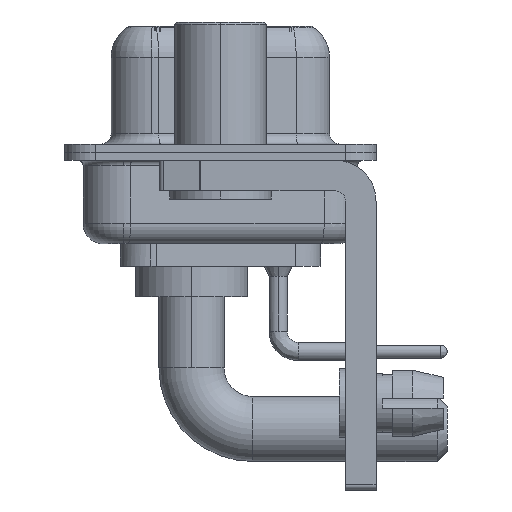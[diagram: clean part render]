
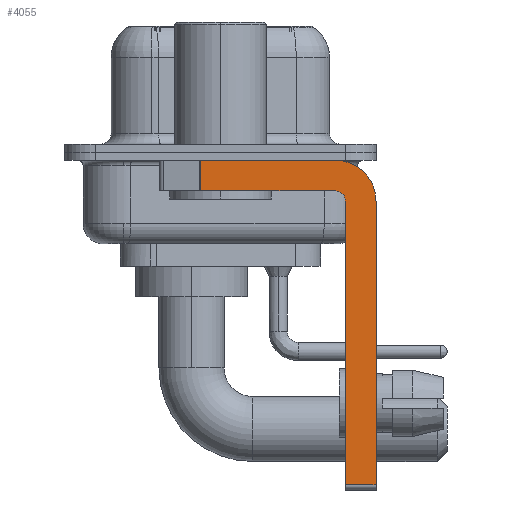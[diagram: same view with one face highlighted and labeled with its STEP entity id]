
A CAD part, left-side view. The second image highlights one B-rep face of the part: STEP entity #4055.
In plain terms, the highlighted planar face has unit normal (-1, 0, 0).
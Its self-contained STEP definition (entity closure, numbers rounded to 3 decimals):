
#403 = CARTESIAN_POINT ( 'NONE',  ( -2.9, -6.15, -16.6 ) ) ;
#712 = LINE ( 'NONE', #10209, #11654 ) ;
#1400 = CIRCLE ( 'NONE', #18189, 2. ) ;
#1860 = CARTESIAN_POINT ( 'NONE',  ( -2.9, 0.978, -0.4 ) ) ;
#1988 = LINE ( 'NONE', #25320, #6661 ) ;
#2259 = VERTEX_POINT ( 'NONE', #6362 ) ;
#2301 = EDGE_CURVE ( 'NONE', #12486, #19635, #712, .T. ) ;
#2708 = DIRECTION ( 'NONE',  ( -1., 0., 0. ) ) ;
#2727 = LINE ( 'NONE', #24270, #3816 ) ;
#2731 = PLANE ( 'NONE',  #23959 ) ;
#2754 = ORIENTED_EDGE ( 'NONE', *, *, #25264, .F. ) ;
#3429 = EDGE_CURVE ( 'NONE', #24635, #15286, #1400, .T. ) ;
#3816 = VECTOR ( 'NONE', #10178, 1000. ) ;
#4055 = ADVANCED_FACE ( 'NONE', ( #19576 ), #2731, .F. ) ;
#5858 = CARTESIAN_POINT ( 'NONE',  ( -2.9, -5.65, -2.4 ) ) ;
#6362 = CARTESIAN_POINT ( 'NONE',  ( -2.9, -5.65, -1.9 ) ) ;
#6596 = EDGE_CURVE ( 'NONE', #2259, #19635, #2727, .T. ) ;
#6661 = VECTOR ( 'NONE', #11464, 1000. ) ;
#7591 = EDGE_LOOP ( 'NONE', ( #2754, #23957, #9406, #24365, #22750, #23461, #15998, #7898 ) ) ;
#7898 = ORIENTED_EDGE ( 'NONE', *, *, #3429, .F. ) ;
#8478 = LINE ( 'NONE', #403, #12207 ) ;
#8719 = DIRECTION ( 'NONE',  ( 0., 0., 1. ) ) ;
#9117 = VERTEX_POINT ( 'NONE', #19627 ) ;
#9406 = ORIENTED_EDGE ( 'NONE', *, *, #6596, .F. ) ;
#9830 = DIRECTION ( 'NONE',  ( 0., 0., -1. ) ) ;
#10178 = DIRECTION ( 'NONE',  ( 0., 1., 0. ) ) ;
#10209 = CARTESIAN_POINT ( 'NONE',  ( -2.9, 0.978, -1.9 ) ) ;
#11200 = LINE ( 'NONE', #16843, #11901 ) ;
#11261 = CIRCLE ( 'NONE', #17821, 0.5 ) ;
#11272 = DIRECTION ( 'NONE',  ( 1., 0., 0. ) ) ;
#11388 = CARTESIAN_POINT ( 'NONE',  ( -2.9, -5.65, -2.4 ) ) ;
#11464 = DIRECTION ( 'NONE',  ( 0., 0., -1. ) ) ;
#11654 = VECTOR ( 'NONE', #14063, 1000. ) ;
#11727 = DIRECTION ( 'NONE',  ( 0., -1., 0. ) ) ;
#11901 = VECTOR ( 'NONE', #19144, 1000. ) ;
#12207 = VECTOR ( 'NONE', #12211, 1000. ) ;
#12211 = DIRECTION ( 'NONE',  ( 0., 0., 1. ) ) ;
#12343 = EDGE_CURVE ( 'NONE', #15286, #22567, #1988, .T. ) ;
#12433 = CARTESIAN_POINT ( 'NONE',  ( -2.9, 0.978, -1.9 ) ) ;
#12486 = VERTEX_POINT ( 'NONE', #1860 ) ;
#14063 = DIRECTION ( 'NONE',  ( 0., 0., -1. ) ) ;
#14295 = DIRECTION ( 'NONE',  ( 1., 0., 0. ) ) ;
#14570 = EDGE_CURVE ( 'NONE', #9117, #2259, #11261, .T. ) ;
#15286 = VERTEX_POINT ( 'NONE', #24312 ) ;
#15998 = ORIENTED_EDGE ( 'NONE', *, *, #12343, .F. ) ;
#16512 = CARTESIAN_POINT ( 'NONE',  ( -2.9, -5.65, -0.4 ) ) ;
#16843 = CARTESIAN_POINT ( 'NONE',  ( -2.9, 3., -0.4 ) ) ;
#16870 = EDGE_CURVE ( 'NONE', #24546, #22567, #17632, .T. ) ;
#17500 = EDGE_CURVE ( 'NONE', #24546, #9117, #8478, .T. ) ;
#17632 = LINE ( 'NONE', #21712, #21162 ) ;
#17821 = AXIS2_PLACEMENT_3D ( 'NONE', #22551, #2708, #8719 ) ;
#18189 = AXIS2_PLACEMENT_3D ( 'NONE', #11388, #11272, #24865 ) ;
#19144 = DIRECTION ( 'NONE',  ( 0., -1., 0. ) ) ;
#19576 = FACE_OUTER_BOUND ( 'NONE', #7591, .T. ) ;
#19627 = CARTESIAN_POINT ( 'NONE',  ( -2.9, -6.15, -2.4 ) ) ;
#19635 = VERTEX_POINT ( 'NONE', #12433 ) ;
#21137 = CARTESIAN_POINT ( 'NONE',  ( -2.9, -7.65, -16.35 ) ) ;
#21162 = VECTOR ( 'NONE', #11727, 1000. ) ;
#21712 = CARTESIAN_POINT ( 'NONE',  ( -2.9, -5.65, -16.35 ) ) ;
#22551 = CARTESIAN_POINT ( 'NONE',  ( -2.9, -5.65, -2.4 ) ) ;
#22567 = VERTEX_POINT ( 'NONE', #21137 ) ;
#22750 = ORIENTED_EDGE ( 'NONE', *, *, #17500, .F. ) ;
#23461 = ORIENTED_EDGE ( 'NONE', *, *, #16870, .T. ) ;
#23818 = CARTESIAN_POINT ( 'NONE',  ( -2.9, -6.15, -16.35 ) ) ;
#23957 = ORIENTED_EDGE ( 'NONE', *, *, #2301, .T. ) ;
#23959 = AXIS2_PLACEMENT_3D ( 'NONE', #5858, #14295, #9830 ) ;
#24270 = CARTESIAN_POINT ( 'NONE',  ( -2.9, -5.65, -1.9 ) ) ;
#24312 = CARTESIAN_POINT ( 'NONE',  ( -2.9, -7.65, -2.4 ) ) ;
#24365 = ORIENTED_EDGE ( 'NONE', *, *, #14570, .F. ) ;
#24546 = VERTEX_POINT ( 'NONE', #23818 ) ;
#24635 = VERTEX_POINT ( 'NONE', #16512 ) ;
#24865 = DIRECTION ( 'NONE',  ( 0., 0., -1. ) ) ;
#25264 = EDGE_CURVE ( 'NONE', #12486, #24635, #11200, .T. ) ;
#25320 = CARTESIAN_POINT ( 'NONE',  ( -2.9, -7.65, -2.4 ) ) ;
